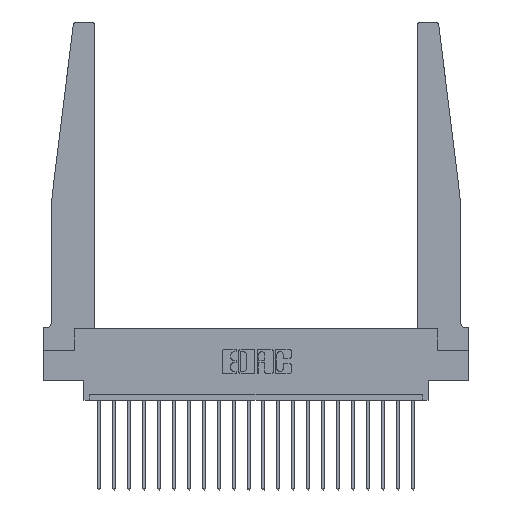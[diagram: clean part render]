
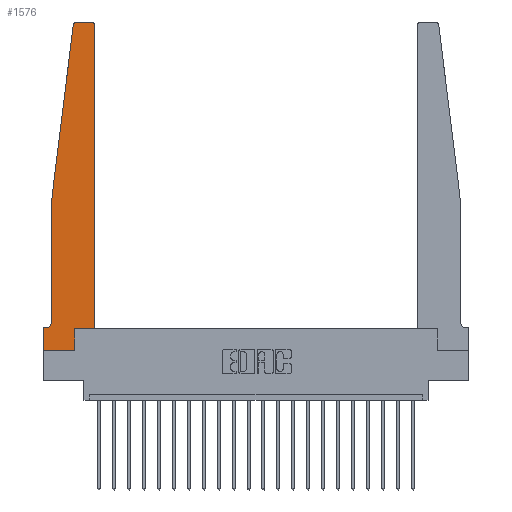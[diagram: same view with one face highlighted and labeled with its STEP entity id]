
A CAD part, top view. The second image highlights one B-rep face of the part: STEP entity #1576.
In plain terms, the highlighted planar face has unit normal (0, 0, 1).
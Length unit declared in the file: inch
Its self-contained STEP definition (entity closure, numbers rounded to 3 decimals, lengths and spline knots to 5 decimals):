
#30 = LINE ( 'NONE', #3879, #17002 ) ;
#83 = LINE ( 'NONE', #20641, #7818 ) ;
#308 = VERTEX_POINT ( 'NONE', #3239 ) ;
#394 = VECTOR ( 'NONE', #8736, 39.37008 ) ;
#403 = VERTEX_POINT ( 'NONE', #18268 ) ;
#488 = CARTESIAN_POINT ( 'NONE',  ( 0.425, 0.18, 0.37 ) ) ;
#867 = CARTESIAN_POINT ( 'NONE',  ( 0., 0., 0.37 ) ) ;
#933 = CARTESIAN_POINT ( 'NONE',  ( 0.27653, 2.72, 0.37 ) ) ;
#1054 = DIRECTION ( 'NONE',  ( 0., 1., 0. ) ) ;
#1180 = ORIENTED_EDGE ( 'NONE', *, *, #6047, .T. ) ;
#1520 = ORIENTED_EDGE ( 'NONE', *, *, #20928, .T. ) ;
#1576 = ADVANCED_FACE ( 'NONE', ( #10226 ), #6533, .T. ) ;
#1985 = LINE ( 'NONE', #14069, #2999 ) ;
#1992 = DIRECTION ( 'NONE',  ( 0., -1., 0. ) ) ;
#2255 = VERTEX_POINT ( 'NONE', #16248 ) ;
#2736 = DIRECTION ( 'NONE',  ( 0., 0., 1. ) ) ;
#2740 = DIRECTION ( 'NONE',  ( 0., -1., 0. ) ) ;
#2880 = CARTESIAN_POINT ( 'NONE',  ( 0.015, 0.2375, 0.37 ) ) ;
#2999 = VECTOR ( 'NONE', #17396, 39.37008 ) ;
#3140 = AXIS2_PLACEMENT_3D ( 'NONE', #16985, #10750, #17857 ) ;
#3239 = CARTESIAN_POINT ( 'NONE',  ( 0., 0., 0.37 ) ) ;
#3312 = LINE ( 'NONE', #867, #20750 ) ;
#3389 = VERTEX_POINT ( 'NONE', #3923 ) ;
#3415 = ORIENTED_EDGE ( 'NONE', *, *, #18821, .T. ) ;
#3797 = LINE ( 'NONE', #19848, #16408 ) ;
#3865 = ORIENTED_EDGE ( 'NONE', *, *, #17120, .T. ) ;
#3879 = CARTESIAN_POINT ( 'NONE',  ( 0., 0., 0.37 ) ) ;
#3923 = CARTESIAN_POINT ( 'NONE',  ( 0.015, 0.1875, 0.37 ) ) ;
#4466 = ORIENTED_EDGE ( 'NONE', *, *, #5344, .T. ) ;
#4769 = VERTEX_POINT ( 'NONE', #7729 ) ;
#4955 = ORIENTED_EDGE ( 'NONE', *, *, #5089, .T. ) ;
#4961 = VERTEX_POINT ( 'NONE', #15229 ) ;
#5089 = EDGE_CURVE ( 'NONE', #12475, #2255, #17846, .T. ) ;
#5344 = EDGE_CURVE ( 'NONE', #403, #13775, #11208, .T. ) ;
#5503 = CIRCLE ( 'NONE', #3140, 0.03 ) ;
#5849 = CARTESIAN_POINT ( 'NONE',  ( 0.425, 0.18, 0.37 ) ) ;
#6028 = DIRECTION ( 'NONE',  ( 1., 0., 0. ) ) ;
#6047 = EDGE_CURVE ( 'NONE', #2255, #4961, #5503, .T. ) ;
#6238 = CARTESIAN_POINT ( 'NONE',  ( 0.27653, 2.75, 0.37 ) ) ;
#6533 = PLANE ( 'NONE',  #10271 ) ;
#6631 = CARTESIAN_POINT ( 'NONE',  ( 0., 0.1875, 0.37 ) ) ;
#6842 = CARTESIAN_POINT ( 'NONE',  ( 0.065, 1.25, 0.37 ) ) ;
#6854 = ORIENTED_EDGE ( 'NONE', *, *, #10345, .T. ) ;
#7549 = CARTESIAN_POINT ( 'NONE',  ( 0., 0.1875, 0.37 ) ) ;
#7729 = CARTESIAN_POINT ( 'NONE',  ( 0.065, 0.2375, 0.37 ) ) ;
#7818 = VECTOR ( 'NONE', #19129, 39.37008 ) ;
#7823 = CARTESIAN_POINT ( 'NONE',  ( 0.24675, 2.72367, 0.37 ) ) ;
#8736 = DIRECTION ( 'NONE',  ( 0., 1., 0. ) ) ;
#9246 = DIRECTION ( 'NONE',  ( 1., 0., 0. ) ) ;
#9263 = LINE ( 'NONE', #19518, #10038 ) ;
#9583 = ORIENTED_EDGE ( 'NONE', *, *, #20588, .T. ) ;
#9738 = DIRECTION ( 'NONE',  ( -1., 0., 0. ) ) ;
#10038 = VECTOR ( 'NONE', #9738, 39.37008 ) ;
#10226 = FACE_OUTER_BOUND ( 'NONE', #15017, .T. ) ;
#10229 = ORIENTED_EDGE ( 'NONE', *, *, #13764, .T. ) ;
#10271 = AXIS2_PLACEMENT_3D ( 'NONE', #6631, #19443, #17940 ) ;
#10345 = EDGE_CURVE ( 'NONE', #3389, #13805, #1985, .T. ) ;
#10623 = VECTOR ( 'NONE', #9246, 39.37008 ) ;
#10749 = EDGE_CURVE ( 'NONE', #15622, #12100, #11781, .T. ) ;
#10750 = DIRECTION ( 'NONE',  ( 0., 0., 1. ) ) ;
#10773 = CARTESIAN_POINT ( 'NONE',  ( 0.2605, 0.18, 0.37 ) ) ;
#11042 = ORIENTED_EDGE ( 'NONE', *, *, #20460, .T. ) ;
#11208 = LINE ( 'NONE', #20257, #394 ) ;
#11781 = CIRCLE ( 'NONE', #16975, 0.03 ) ;
#12019 = DIRECTION ( 'NONE',  ( 1., 0., 0. ) ) ;
#12100 = VERTEX_POINT ( 'NONE', #7823 ) ;
#12475 = VERTEX_POINT ( 'NONE', #13649 ) ;
#13026 = VECTOR ( 'NONE', #1054, 39.37008 ) ;
#13649 = CARTESIAN_POINT ( 'NONE',  ( 0.425, 0.18, 0.37 ) ) ;
#13764 = EDGE_CURVE ( 'NONE', #12100, #18759, #83, .T. ) ;
#13775 = VERTEX_POINT ( 'NONE', #10773 ) ;
#13805 = VERTEX_POINT ( 'NONE', #7549 ) ;
#14069 = CARTESIAN_POINT ( 'NONE',  ( 0.065, 0.1875, 0.37 ) ) ;
#14238 = AXIS2_PLACEMENT_3D ( 'NONE', #2880, #21075, #19426 ) ;
#14971 = EDGE_CURVE ( 'NONE', #13775, #12475, #15261, .T. ) ;
#15017 = EDGE_LOOP ( 'NONE', ( #3865, #15804, #10229, #1520, #9583, #6854, #11042, #3415, #4466, #16755, #4955, #1180 ) ) ;
#15229 = CARTESIAN_POINT ( 'NONE',  ( 0.395, 2.75, 0.37 ) ) ;
#15261 = LINE ( 'NONE', #5849, #10623 ) ;
#15622 = VERTEX_POINT ( 'NONE', #6238 ) ;
#15804 = ORIENTED_EDGE ( 'NONE', *, *, #10749, .T. ) ;
#16248 = CARTESIAN_POINT ( 'NONE',  ( 0.425, 2.72, 0.37 ) ) ;
#16408 = VECTOR ( 'NONE', #1992, 39.37008 ) ;
#16755 = ORIENTED_EDGE ( 'NONE', *, *, #14971, .T. ) ;
#16975 = AXIS2_PLACEMENT_3D ( 'NONE', #933, #2736, #6028 ) ;
#16985 = CARTESIAN_POINT ( 'NONE',  ( 0.395, 2.72, 0.37 ) ) ;
#17002 = VECTOR ( 'NONE', #12019, 39.37008 ) ;
#17120 = EDGE_CURVE ( 'NONE', #4961, #15622, #9263, .T. ) ;
#17396 = DIRECTION ( 'NONE',  ( -1., 0., 0. ) ) ;
#17846 = LINE ( 'NONE', #488, #13026 ) ;
#17857 = DIRECTION ( 'NONE',  ( 1., 0., 0. ) ) ;
#17940 = DIRECTION ( 'NONE',  ( 1., 0., 0. ) ) ;
#18268 = CARTESIAN_POINT ( 'NONE',  ( 0.2605, 0., 0.37 ) ) ;
#18759 = VERTEX_POINT ( 'NONE', #6842 ) ;
#18821 = EDGE_CURVE ( 'NONE', #308, #403, #30, .T. ) ;
#19129 = DIRECTION ( 'NONE',  ( -0.122, -0.992, 0. ) ) ;
#19204 = CIRCLE ( 'NONE', #14238, 0.05 ) ;
#19426 = DIRECTION ( 'NONE',  ( -1., 0., 0. ) ) ;
#19443 = DIRECTION ( 'NONE',  ( 0., 0., 1. ) ) ;
#19518 = CARTESIAN_POINT ( 'NONE',  ( 0.25, 2.75, 0.37 ) ) ;
#19848 = CARTESIAN_POINT ( 'NONE',  ( 0.065, 1.25, 0.37 ) ) ;
#20257 = CARTESIAN_POINT ( 'NONE',  ( 0.2605, 0.18, 0.37 ) ) ;
#20460 = EDGE_CURVE ( 'NONE', #13805, #308, #3312, .T. ) ;
#20588 = EDGE_CURVE ( 'NONE', #4769, #3389, #19204, .T. ) ;
#20641 = CARTESIAN_POINT ( 'NONE',  ( 0.065, 1.25, 0.37 ) ) ;
#20750 = VECTOR ( 'NONE', #2740, 39.37008 ) ;
#20928 = EDGE_CURVE ( 'NONE', #18759, #4769, #3797, .T. ) ;
#21075 = DIRECTION ( 'NONE',  ( 0., 0., -1. ) ) ;
